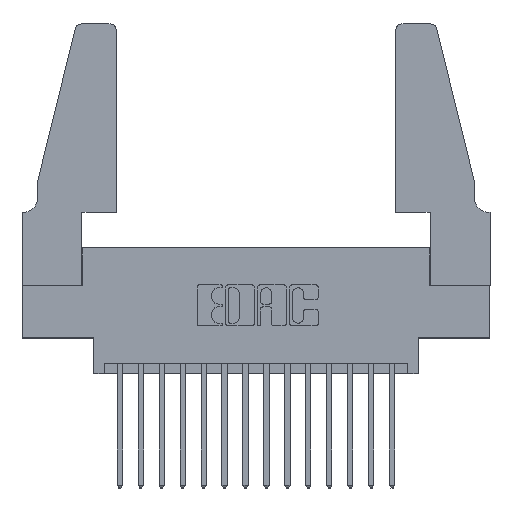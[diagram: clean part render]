
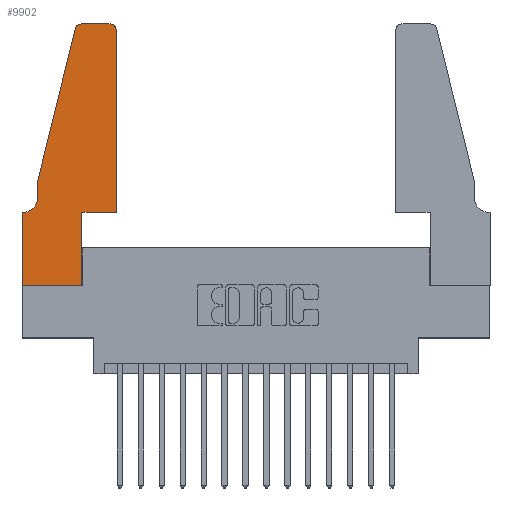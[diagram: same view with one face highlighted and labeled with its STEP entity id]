
A CAD part, top view. The second image highlights one B-rep face of the part: STEP entity #9902.
In plain terms, the highlighted planar face has unit normal (0, 0, 1).
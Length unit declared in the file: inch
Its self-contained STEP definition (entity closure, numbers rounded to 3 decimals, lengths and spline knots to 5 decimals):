
#75 = CARTESIAN_POINT ( 'NONE',  ( 0.4505, 0.35, 0.37 ) ) ;
#179 = ORIENTED_EDGE ( 'NONE', *, *, #12803, .T. ) ;
#436 = LINE ( 'NONE', #8277, #843 ) ;
#530 = DIRECTION ( 'NONE',  ( -1., 0., 0. ) ) ;
#640 = CARTESIAN_POINT ( 'NONE',  ( 0., 0.35, 0.37 ) ) ;
#716 = LINE ( 'NONE', #11146, #5444 ) ;
#784 = VERTEX_POINT ( 'NONE', #14545 ) ;
#788 = VERTEX_POINT ( 'NONE', #5149 ) ;
#843 = VECTOR ( 'NONE', #9416, 39.37008 ) ;
#1006 = DIRECTION ( 'NONE',  ( 0., 0., 1. ) ) ;
#1277 = CARTESIAN_POINT ( 'NONE',  ( 0.4505, 0.35, 0.37 ) ) ;
#1448 = CARTESIAN_POINT ( 'NONE',  ( 0., 0.35, 0.37 ) ) ;
#1511 = CARTESIAN_POINT ( 'NONE',  ( 0.0755, 0.35, 0.37 ) ) ;
#1687 = AXIS2_PLACEMENT_3D ( 'NONE', #640, #8513, #13776 ) ;
#1793 = ORIENTED_EDGE ( 'NONE', *, *, #13189, .T. ) ;
#1932 = VECTOR ( 'NONE', #7860, 39.37008 ) ;
#2273 = LINE ( 'NONE', #8394, #7191 ) ;
#2433 = ORIENTED_EDGE ( 'NONE', *, *, #7184, .T. ) ;
#2886 = LINE ( 'NONE', #13725, #9242 ) ;
#3415 = DIRECTION ( 'NONE',  ( 0., 1., 0. ) ) ;
#3657 = CARTESIAN_POINT ( 'NONE',  ( 0.284, 1.22, 0.37 ) ) ;
#3848 = VERTEX_POINT ( 'NONE', #15342 ) ;
#3984 = CIRCLE ( 'NONE', #15617, 0.07 ) ;
#4515 = DIRECTION ( 'NONE',  ( 0., 0., -1. ) ) ;
#4947 = FACE_OUTER_BOUND ( 'NONE', #6362, .T. ) ;
#5010 = CARTESIAN_POINT ( 'NONE',  ( 0.0755, 0.5, 0.37 ) ) ;
#5041 = AXIS2_PLACEMENT_3D ( 'NONE', #7411, #8656, #9856 ) ;
#5149 = CARTESIAN_POINT ( 'NONE',  ( 0.284, 1.25, 0.37 ) ) ;
#5209 = CARTESIAN_POINT ( 'NONE',  ( 0.2865, 0.35, 0.37 ) ) ;
#5444 = VECTOR ( 'NONE', #15155, 39.37008 ) ;
#5544 = ORIENTED_EDGE ( 'NONE', *, *, #9875, .T. ) ;
#5557 = VECTOR ( 'NONE', #14123, 39.37008 ) ;
#5686 = ORIENTED_EDGE ( 'NONE', *, *, #14368, .T. ) ;
#6211 = VERTEX_POINT ( 'NONE', #5209 ) ;
#6352 = VECTOR ( 'NONE', #12140, 39.37008 ) ;
#6362 = EDGE_LOOP ( 'NONE', ( #11896, #16931, #1793, #6509, #15825, #6531, #9991, #2433, #14875, #179, #5544, #5686 ) ) ;
#6509 = ORIENTED_EDGE ( 'NONE', *, *, #14474, .T. ) ;
#6531 = ORIENTED_EDGE ( 'NONE', *, *, #15356, .T. ) ;
#6816 = EDGE_CURVE ( 'NONE', #16383, #11808, #3984, .T. ) ;
#6925 = CARTESIAN_POINT ( 'NONE',  ( 0., 0., 0.37 ) ) ;
#7132 = VERTEX_POINT ( 'NONE', #1448 ) ;
#7184 = EDGE_CURVE ( 'NONE', #8343, #7389, #716, .T. ) ;
#7191 = VECTOR ( 'NONE', #530, 39.37008 ) ;
#7389 = VERTEX_POINT ( 'NONE', #11542 ) ;
#7411 = CARTESIAN_POINT ( 'NONE',  ( 0.4205, 1.22, 0.37 ) ) ;
#7860 = DIRECTION ( 'NONE',  ( 1., 0., 0. ) ) ;
#8025 = EDGE_CURVE ( 'NONE', #788, #12739, #16132, .T. ) ;
#8205 = EDGE_CURVE ( 'NONE', #7389, #6211, #16336, .T. ) ;
#8277 = CARTESIAN_POINT ( 'NONE',  ( 0., 0., 0.37 ) ) ;
#8343 = VERTEX_POINT ( 'NONE', #6925 ) ;
#8370 = EDGE_CURVE ( 'NONE', #7132, #8343, #436, .T. ) ;
#8394 = CARTESIAN_POINT ( 'NONE',  ( 0.2605, 1.25, 0.37 ) ) ;
#8513 = DIRECTION ( 'NONE',  ( 0., 0., 1. ) ) ;
#8611 = LINE ( 'NONE', #5010, #5557 ) ;
#8656 = DIRECTION ( 'NONE',  ( 0., 0., 1. ) ) ;
#8785 = LINE ( 'NONE', #1511, #6352 ) ;
#9032 = CARTESIAN_POINT ( 'NONE',  ( 0.0755, 0.5, 0.37 ) ) ;
#9242 = VECTOR ( 'NONE', #3415, 39.37008 ) ;
#9416 = DIRECTION ( 'NONE',  ( 0., -1., 0. ) ) ;
#9544 = VERTEX_POINT ( 'NONE', #75 ) ;
#9856 = DIRECTION ( 'NONE',  ( 1., 0., 0. ) ) ;
#9875 = EDGE_CURVE ( 'NONE', #9544, #3848, #2886, .T. ) ;
#9902 = ADVANCED_FACE ( 'NONE', ( #4947 ), #12461, .T. ) ;
#9925 = EDGE_CURVE ( 'NONE', #784, #788, #2273, .T. ) ;
#9991 = ORIENTED_EDGE ( 'NONE', *, *, #8370, .T. ) ;
#10060 = CARTESIAN_POINT ( 'NONE',  ( 0.0055, 0.35, 0.37 ) ) ;
#10068 = CARTESIAN_POINT ( 'NONE',  ( 0.0755, 0.5, 0.37 ) ) ;
#10427 = CARTESIAN_POINT ( 'NONE',  ( 0.2865, 0.35, 0.37 ) ) ;
#10956 = AXIS2_PLACEMENT_3D ( 'NONE', #3657, #1006, #15537 ) ;
#10991 = CARTESIAN_POINT ( 'NONE',  ( 0.0755, 0.42, 0.37 ) ) ;
#11146 = CARTESIAN_POINT ( 'NONE',  ( 0., 0., 0.37 ) ) ;
#11542 = CARTESIAN_POINT ( 'NONE',  ( 0.2865, 0., 0.37 ) ) ;
#11808 = VERTEX_POINT ( 'NONE', #10060 ) ;
#11896 = ORIENTED_EDGE ( 'NONE', *, *, #9925, .T. ) ;
#11946 = VERTEX_POINT ( 'NONE', #9032 ) ;
#12140 = DIRECTION ( 'NONE',  ( -1., 0., 0. ) ) ;
#12231 = LINE ( 'NONE', #1277, #1932 ) ;
#12381 = CARTESIAN_POINT ( 'NONE',  ( 0.0055, 0.42, 0.37 ) ) ;
#12461 = PLANE ( 'NONE',  #1687 ) ;
#12739 = VERTEX_POINT ( 'NONE', #14456 ) ;
#12803 = EDGE_CURVE ( 'NONE', #6211, #9544, #12231, .T. ) ;
#13094 = DIRECTION ( 'NONE',  ( 0., 1., 0. ) ) ;
#13189 = EDGE_CURVE ( 'NONE', #12739, #11946, #15128, .T. ) ;
#13421 = VECTOR ( 'NONE', #13094, 39.37008 ) ;
#13716 = DIRECTION ( 'NONE',  ( -1., 0., 0. ) ) ;
#13725 = CARTESIAN_POINT ( 'NONE',  ( 0.4505, 0.35, 0.37 ) ) ;
#13776 = DIRECTION ( 'NONE',  ( 1., 0., 0. ) ) ;
#14037 = DIRECTION ( 'NONE',  ( -0.239, -0.971, 0. ) ) ;
#14123 = DIRECTION ( 'NONE',  ( 0., -1., 0. ) ) ;
#14368 = EDGE_CURVE ( 'NONE', #3848, #784, #16906, .T. ) ;
#14456 = CARTESIAN_POINT ( 'NONE',  ( 0.25487, 1.22718, 0.37 ) ) ;
#14474 = EDGE_CURVE ( 'NONE', #11946, #16383, #8611, .T. ) ;
#14545 = CARTESIAN_POINT ( 'NONE',  ( 0.4205, 1.25, 0.37 ) ) ;
#14875 = ORIENTED_EDGE ( 'NONE', *, *, #8205, .T. ) ;
#14916 = VECTOR ( 'NONE', #14037, 39.37008 ) ;
#15128 = LINE ( 'NONE', #10068, #14916 ) ;
#15155 = DIRECTION ( 'NONE',  ( 1., 0., 0. ) ) ;
#15342 = CARTESIAN_POINT ( 'NONE',  ( 0.4505, 1.22, 0.37 ) ) ;
#15356 = EDGE_CURVE ( 'NONE', #11808, #7132, #8785, .T. ) ;
#15537 = DIRECTION ( 'NONE',  ( 1., 0., 0. ) ) ;
#15617 = AXIS2_PLACEMENT_3D ( 'NONE', #12381, #4515, #13716 ) ;
#15825 = ORIENTED_EDGE ( 'NONE', *, *, #6816, .T. ) ;
#16132 = CIRCLE ( 'NONE', #10956, 0.03 ) ;
#16336 = LINE ( 'NONE', #10427, #13421 ) ;
#16383 = VERTEX_POINT ( 'NONE', #10991 ) ;
#16906 = CIRCLE ( 'NONE', #5041, 0.03 ) ;
#16931 = ORIENTED_EDGE ( 'NONE', *, *, #8025, .T. ) ;
